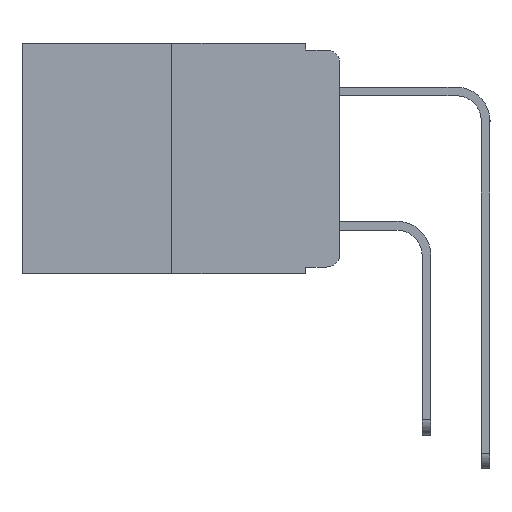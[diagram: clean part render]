
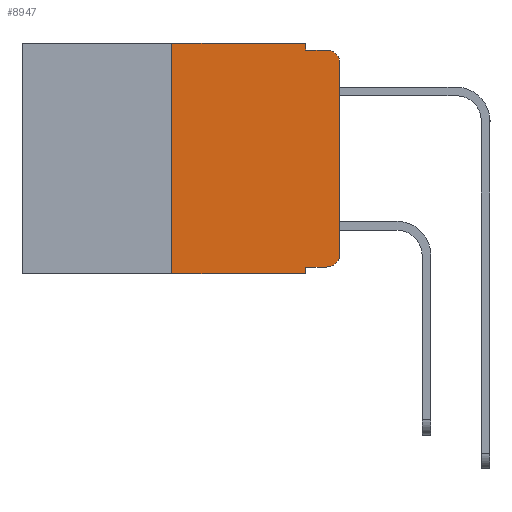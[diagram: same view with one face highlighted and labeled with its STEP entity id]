
A CAD part, left-side view. The second image highlights one B-rep face of the part: STEP entity #8947.
In plain terms, the highlighted planar face has unit normal (-1, 0, 0).
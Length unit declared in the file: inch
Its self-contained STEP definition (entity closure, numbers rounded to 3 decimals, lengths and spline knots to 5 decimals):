
#247 = CARTESIAN_POINT ( 'NONE',  ( 0., 0.051, 0. ) ) ;
#487 = VERTEX_POINT ( 'NONE', #13000 ) ;
#617 = DIRECTION ( 'NONE',  ( 0., -1., 0. ) ) ;
#619 = VERTEX_POINT ( 'NONE', #10731 ) ;
#646 = LINE ( 'NONE', #3888, #8314 ) ;
#756 = CARTESIAN_POINT ( 'NONE',  ( 0., 0.051, -0.333 ) ) ;
#833 = DIRECTION ( 'NONE',  ( -1., 0., 0. ) ) ;
#845 = CARTESIAN_POINT ( 'NONE',  ( 0., 0.25, -0.343 ) ) ;
#1136 = DIRECTION ( 'NONE',  ( 0., -1., 0. ) ) ;
#1244 = CARTESIAN_POINT ( 'NONE',  ( 0., 0.02, -0.313 ) ) ;
#1283 = DIRECTION ( 'NONE',  ( 0., 0., -1. ) ) ;
#1445 = DIRECTION ( 'NONE',  ( 0., -1., 0. ) ) ;
#1452 = EDGE_CURVE ( 'NONE', #2693, #487, #2273, .T. ) ;
#1569 = VERTEX_POINT ( 'NONE', #2196 ) ;
#1578 = DIRECTION ( 'NONE',  ( 0., 0., 1. ) ) ;
#1716 = EDGE_CURVE ( 'NONE', #619, #1569, #2435, .T. ) ;
#1909 = DIRECTION ( 'NONE',  ( 0., 0., -1. ) ) ;
#2184 = VECTOR ( 'NONE', #1578, 39.37008 ) ;
#2196 = CARTESIAN_POINT ( 'NONE',  ( 0., 0., -0.313 ) ) ;
#2273 = CIRCLE ( 'NONE', #10441, 0.02 ) ;
#2334 = VERTEX_POINT ( 'NONE', #2843 ) ;
#2349 = DIRECTION ( 'NONE',  ( 0., 0., 1. ) ) ;
#2435 = CIRCLE ( 'NONE', #9507, 0.02 ) ;
#2693 = VERTEX_POINT ( 'NONE', #3763 ) ;
#2781 = PLANE ( 'NONE',  #11691 ) ;
#2843 = CARTESIAN_POINT ( 'NONE',  ( 0., 0.051, 0. ) ) ;
#2874 = DIRECTION ( 'NONE',  ( 0., -1., 0. ) ) ;
#2881 = EDGE_CURVE ( 'NONE', #1569, #2693, #3840, .T. ) ;
#3202 = VERTEX_POINT ( 'NONE', #845 ) ;
#3763 = CARTESIAN_POINT ( 'NONE',  ( 0., 0., -0.03 ) ) ;
#3822 = CARTESIAN_POINT ( 'NONE',  ( 0., 0.473, 0. ) ) ;
#3840 = LINE ( 'NONE', #8789, #2184 ) ;
#3849 = EDGE_CURVE ( 'NONE', #10027, #619, #11346, .T. ) ;
#3888 = CARTESIAN_POINT ( 'NONE',  ( 0., 0.051, -0.01 ) ) ;
#4316 = ORIENTED_EDGE ( 'NONE', *, *, #3849, .T. ) ;
#4870 = VECTOR ( 'NONE', #1136, 39.37008 ) ;
#4887 = DIRECTION ( 'NONE',  ( 0., 0., -1. ) ) ;
#4965 = VECTOR ( 'NONE', #617, 39.37008 ) ;
#5347 = ORIENTED_EDGE ( 'NONE', *, *, #7110, .F. ) ;
#5757 = ORIENTED_EDGE ( 'NONE', *, *, #6655, .F. ) ;
#6054 = LINE ( 'NONE', #9114, #8422 ) ;
#6109 = VERTEX_POINT ( 'NONE', #9077 ) ;
#6360 = LINE ( 'NONE', #247, #11412 ) ;
#6466 = ORIENTED_EDGE ( 'NONE', *, *, #1716, .T. ) ;
#6655 = EDGE_CURVE ( 'NONE', #10027, #12290, #6054, .T. ) ;
#6837 = VECTOR ( 'NONE', #2349, 39.37008 ) ;
#6893 = EDGE_LOOP ( 'NONE', ( #12281, #8045, #10926, #7755, #5347, #9099, #12843, #5757, #4316, #6466 ) ) ;
#7110 = EDGE_CURVE ( 'NONE', #9349, #2334, #8411, .T. ) ;
#7517 = DIRECTION ( 'NONE',  ( -1., 0., 0. ) ) ;
#7526 = CARTESIAN_POINT ( 'NONE',  ( 0., 0.25, 0. ) ) ;
#7592 = LINE ( 'NONE', #7982, #4870 ) ;
#7755 = ORIENTED_EDGE ( 'NONE', *, *, #10028, .F. ) ;
#7982 = CARTESIAN_POINT ( 'NONE',  ( 0., 0.473, -0.343 ) ) ;
#8045 = ORIENTED_EDGE ( 'NONE', *, *, #1452, .T. ) ;
#8096 = VECTOR ( 'NONE', #1445, 39.37008 ) ;
#8314 = VECTOR ( 'NONE', #2874, 39.37008 ) ;
#8340 = EDGE_CURVE ( 'NONE', #3202, #12290, #7592, .T. ) ;
#8361 = FACE_OUTER_BOUND ( 'NONE', #6893, .T. ) ;
#8411 = LINE ( 'NONE', #12247, #8096 ) ;
#8422 = VECTOR ( 'NONE', #8975, 39.37008 ) ;
#8526 = DIRECTION ( 'NONE',  ( 0., 0., -1. ) ) ;
#8534 = CARTESIAN_POINT ( 'NONE',  ( 0., 0.25, 0. ) ) ;
#8789 = CARTESIAN_POINT ( 'NONE',  ( 0., 0., 0. ) ) ;
#8892 = LINE ( 'NONE', #8534, #6837 ) ;
#8947 = ADVANCED_FACE ( 'NONE', ( #8361 ), #2781, .F. ) ;
#8975 = DIRECTION ( 'NONE',  ( 0., 0., -1. ) ) ;
#9077 = CARTESIAN_POINT ( 'NONE',  ( 0., 0.051, -0.01 ) ) ;
#9099 = ORIENTED_EDGE ( 'NONE', *, *, #9342, .F. ) ;
#9114 = CARTESIAN_POINT ( 'NONE',  ( 0., 0.051, 0. ) ) ;
#9342 = EDGE_CURVE ( 'NONE', #3202, #9349, #8892, .T. ) ;
#9349 = VERTEX_POINT ( 'NONE', #7526 ) ;
#9507 = AXIS2_PLACEMENT_3D ( 'NONE', #1244, #7517, #8526 ) ;
#10027 = VERTEX_POINT ( 'NONE', #12557 ) ;
#10028 = EDGE_CURVE ( 'NONE', #2334, #6109, #6360, .T. ) ;
#10441 = AXIS2_PLACEMENT_3D ( 'NONE', #12092, #833, #1909 ) ;
#10731 = CARTESIAN_POINT ( 'NONE',  ( 0., 0.02, -0.333 ) ) ;
#10926 = ORIENTED_EDGE ( 'NONE', *, *, #12693, .F. ) ;
#10993 = DIRECTION ( 'NONE',  ( 1., 0., 0. ) ) ;
#11346 = LINE ( 'NONE', #756, #4965 ) ;
#11372 = CARTESIAN_POINT ( 'NONE',  ( 0., 0.051, -0.343 ) ) ;
#11412 = VECTOR ( 'NONE', #1283, 39.37008 ) ;
#11691 = AXIS2_PLACEMENT_3D ( 'NONE', #3822, #10993, #4887 ) ;
#12092 = CARTESIAN_POINT ( 'NONE',  ( 0., 0.02, -0.03 ) ) ;
#12247 = CARTESIAN_POINT ( 'NONE',  ( 0., 0.473, 0. ) ) ;
#12281 = ORIENTED_EDGE ( 'NONE', *, *, #2881, .T. ) ;
#12290 = VERTEX_POINT ( 'NONE', #11372 ) ;
#12557 = CARTESIAN_POINT ( 'NONE',  ( 0., 0.051, -0.333 ) ) ;
#12693 = EDGE_CURVE ( 'NONE', #6109, #487, #646, .T. ) ;
#12843 = ORIENTED_EDGE ( 'NONE', *, *, #8340, .T. ) ;
#13000 = CARTESIAN_POINT ( 'NONE',  ( 0., 0.02, -0.01 ) ) ;
